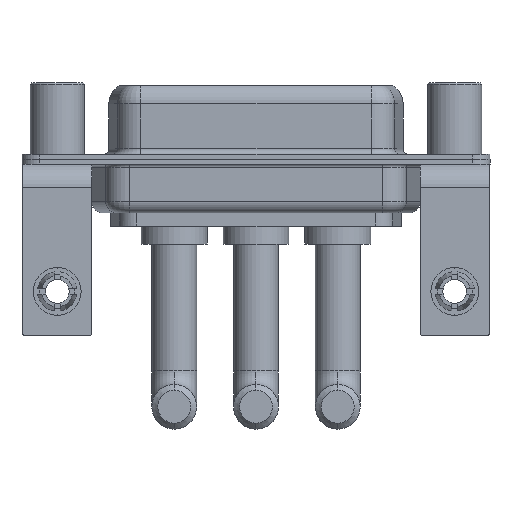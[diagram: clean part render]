
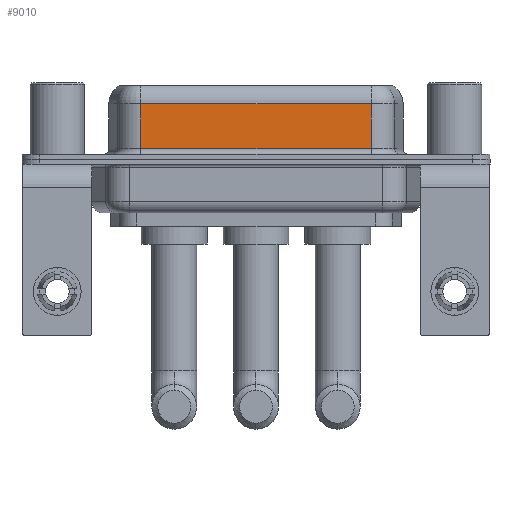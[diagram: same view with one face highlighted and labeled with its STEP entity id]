
A CAD part, front view. The second image highlights one B-rep face of the part: STEP entity #9010.
In plain terms, the highlighted planar face has unit normal (0, -1, 0).
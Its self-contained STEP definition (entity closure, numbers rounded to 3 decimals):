
#156 = VECTOR ( 'NONE', #16042, 1000. ) ;
#667 = DIRECTION ( 'NONE',  ( 0., 0., -1. ) ) ;
#882 = DIRECTION ( 'NONE',  ( 0., 0., 1. ) ) ;
#1100 = ORIENTED_EDGE ( 'NONE', *, *, #10210, .T. ) ;
#1152 = VECTOR ( 'NONE', #12066, 1000. ) ;
#2924 = CARTESIAN_POINT ( 'NONE',  ( 7.013, -3.95, 6.4 ) ) ;
#2978 = VECTOR ( 'NONE', #667, 1000. ) ;
#3470 = FACE_OUTER_BOUND ( 'NONE', #11003, .T. ) ;
#3577 = CARTESIAN_POINT ( 'NONE',  ( 26.287, -3.95, 0.9 ) ) ;
#4040 = VECTOR ( 'NONE', #9974, 1000. ) ;
#4528 = LINE ( 'NONE', #9609, #156 ) ;
#4670 = VERTEX_POINT ( 'NONE', #8937 ) ;
#6381 = VERTEX_POINT ( 'NONE', #3577 ) ;
#6925 = EDGE_CURVE ( 'NONE', #12590, #4670, #13554, .T. ) ;
#6973 = LINE ( 'NONE', #15914, #1152 ) ;
#7384 = CARTESIAN_POINT ( 'NONE',  ( 26.287, -3.95, 4.65 ) ) ;
#8408 = EDGE_CURVE ( 'NONE', #4670, #14876, #13250, .T. ) ;
#8937 = CARTESIAN_POINT ( 'NONE',  ( 7.013, -3.95, 4.65 ) ) ;
#9010 = ADVANCED_FACE ( 'NONE', ( #3470 ), #11056, .F. ) ;
#9479 = ORIENTED_EDGE ( 'NONE', *, *, #8408, .T. ) ;
#9609 = CARTESIAN_POINT ( 'NONE',  ( 26.287, -3.95, 6.4 ) ) ;
#9833 = ORIENTED_EDGE ( 'NONE', *, *, #6925, .T. ) ;
#9974 = DIRECTION ( 'NONE',  ( -1., 0., 0. ) ) ;
#10210 = EDGE_CURVE ( 'NONE', #14876, #6381, #6973, .T. ) ;
#10441 = AXIS2_PLACEMENT_3D ( 'NONE', #14885, #13474, #882 ) ;
#11003 = EDGE_LOOP ( 'NONE', ( #12498, #9833, #9479, #1100 ) ) ;
#11056 = PLANE ( 'NONE',  #10441 ) ;
#12066 = DIRECTION ( 'NONE',  ( 1., 0., 0. ) ) ;
#12498 = ORIENTED_EDGE ( 'NONE', *, *, #14039, .F. ) ;
#12590 = VERTEX_POINT ( 'NONE', #13034 ) ;
#13034 = CARTESIAN_POINT ( 'NONE',  ( 26.287, -3.95, 4.65 ) ) ;
#13250 = LINE ( 'NONE', #2924, #2978 ) ;
#13474 = DIRECTION ( 'NONE',  ( 0., 1., 0. ) ) ;
#13554 = LINE ( 'NONE', #7384, #4040 ) ;
#14039 = EDGE_CURVE ( 'NONE', #12590, #6381, #4528, .T. ) ;
#14876 = VERTEX_POINT ( 'NONE', #15509 ) ;
#14885 = CARTESIAN_POINT ( 'NONE',  ( 26.287, -3.95, 6.4 ) ) ;
#15509 = CARTESIAN_POINT ( 'NONE',  ( 7.013, -3.95, 0.9 ) ) ;
#15914 = CARTESIAN_POINT ( 'NONE',  ( 26.287, -3.95, 0.9 ) ) ;
#16042 = DIRECTION ( 'NONE',  ( 0., 0., -1. ) ) ;
